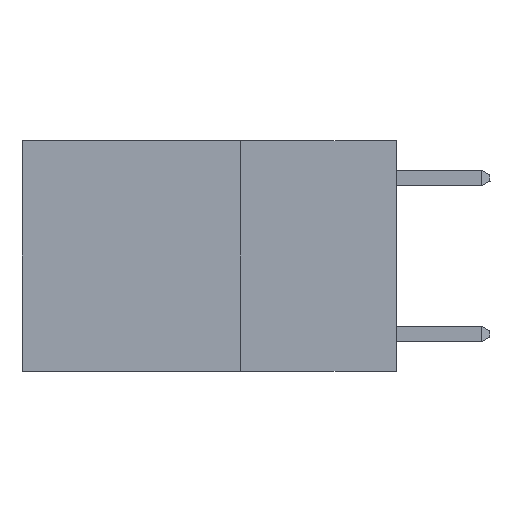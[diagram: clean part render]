
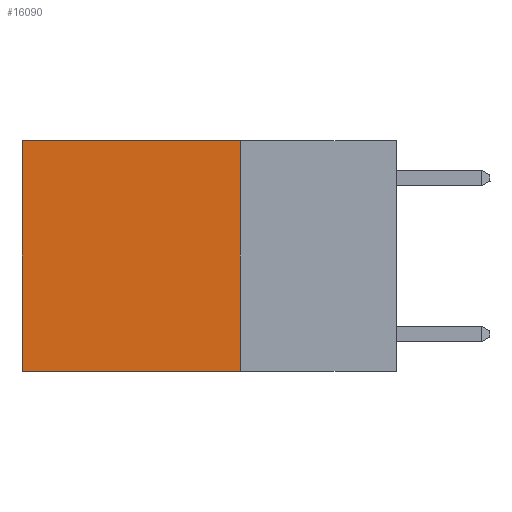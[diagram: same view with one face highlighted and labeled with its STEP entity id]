
A CAD part, left-side view. The second image highlights one B-rep face of the part: STEP entity #16090.
In plain terms, the highlighted planar face has unit normal (-1, 0, 0).
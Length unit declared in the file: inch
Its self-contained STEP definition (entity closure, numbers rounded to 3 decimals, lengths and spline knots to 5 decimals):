
#353 = DIRECTION ( 'NONE',  ( 1., 0., 0. ) ) ;
#703 = LINE ( 'NONE', #16689, #5195 ) ;
#955 = CARTESIAN_POINT ( 'NONE',  ( 0.2625, 0.25, 0. ) ) ;
#1216 = CARTESIAN_POINT ( 'NONE',  ( 0.2625, 0.25, -0.37 ) ) ;
#1829 = EDGE_CURVE ( 'NONE', #7219, #23823, #11768, .T. ) ;
#5195 = VECTOR ( 'NONE', #26060, 39.37008 ) ;
#6813 = CARTESIAN_POINT ( 'NONE',  ( 0.2625, 0.6, -0.37 ) ) ;
#7219 = VERTEX_POINT ( 'NONE', #1216 ) ;
#8675 = CARTESIAN_POINT ( 'NONE',  ( 0.2625, 0.25, 0. ) ) ;
#9418 = DIRECTION ( 'NONE',  ( 0., 1., 0. ) ) ;
#9489 = CARTESIAN_POINT ( 'NONE',  ( 0.2625, 0.25, -0.37 ) ) ;
#9502 = PLANE ( 'NONE',  #23749 ) ;
#9929 = CARTESIAN_POINT ( 'NONE',  ( 0.2625, 0.25, 0. ) ) ;
#11768 = LINE ( 'NONE', #9489, #19664 ) ;
#12447 = VECTOR ( 'NONE', #9418, 39.37008 ) ;
#14029 = LINE ( 'NONE', #19084, #28316 ) ;
#14152 = DIRECTION ( 'NONE',  ( 0., 0., -1. ) ) ;
#14329 = VERTEX_POINT ( 'NONE', #30843 ) ;
#14340 = DIRECTION ( 'NONE',  ( 0., 1., 0. ) ) ;
#14550 = EDGE_CURVE ( 'NONE', #17103, #14329, #22189, .T. ) ;
#15078 = ORIENTED_EDGE ( 'NONE', *, *, #27552, .F. ) ;
#16009 = ORIENTED_EDGE ( 'NONE', *, *, #22368, .T. ) ;
#16090 = ADVANCED_FACE ( 'NONE', ( #22466 ), #9502, .F. ) ;
#16689 = CARTESIAN_POINT ( 'NONE',  ( 0.2625, 0.25, 0. ) ) ;
#17103 = VERTEX_POINT ( 'NONE', #955 ) ;
#19084 = CARTESIAN_POINT ( 'NONE',  ( 0.2625, 0.6, 0. ) ) ;
#19188 = ORIENTED_EDGE ( 'NONE', *, *, #14550, .T. ) ;
#19664 = VECTOR ( 'NONE', #14340, 39.37008 ) ;
#22189 = LINE ( 'NONE', #8675, #12447 ) ;
#22368 = EDGE_CURVE ( 'NONE', #14329, #23823, #14029, .T. ) ;
#22466 = FACE_OUTER_BOUND ( 'NONE', #24172, .T. ) ;
#23749 = AXIS2_PLACEMENT_3D ( 'NONE', #9929, #353, #24450 ) ;
#23823 = VERTEX_POINT ( 'NONE', #6813 ) ;
#24172 = EDGE_LOOP ( 'NONE', ( #16009, #28449, #15078, #19188 ) ) ;
#24450 = DIRECTION ( 'NONE',  ( 0., 0., -1. ) ) ;
#26060 = DIRECTION ( 'NONE',  ( 0., 0., -1. ) ) ;
#27552 = EDGE_CURVE ( 'NONE', #17103, #7219, #703, .T. ) ;
#28316 = VECTOR ( 'NONE', #14152, 39.37008 ) ;
#28449 = ORIENTED_EDGE ( 'NONE', *, *, #1829, .F. ) ;
#30843 = CARTESIAN_POINT ( 'NONE',  ( 0.2625, 0.6, 0. ) ) ;
